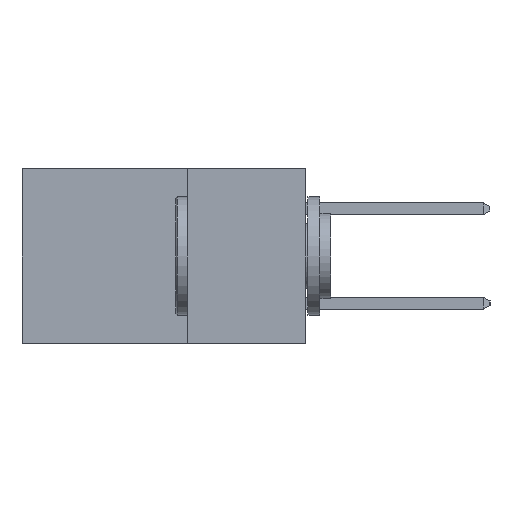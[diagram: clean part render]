
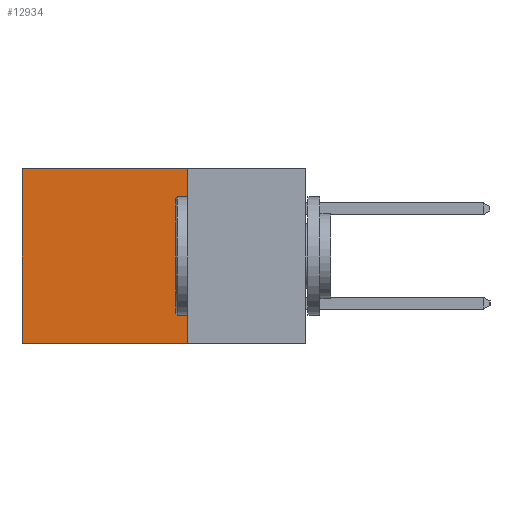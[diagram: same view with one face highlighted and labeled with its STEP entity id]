
A CAD part, left-side view. The second image highlights one B-rep face of the part: STEP entity #12934.
In plain terms, the highlighted planar face has unit normal (-1, 0, 0).
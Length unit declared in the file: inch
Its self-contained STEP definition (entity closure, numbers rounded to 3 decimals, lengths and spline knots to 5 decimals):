
#339 = EDGE_CURVE ( 'NONE', #3913, #16367, #9802, .T. ) ;
#655 = EDGE_LOOP ( 'NONE', ( #7367, #7930, #14706, #15632 ) ) ;
#988 = LINE ( 'NONE', #4701, #7487 ) ;
#1065 = PLANE ( 'NONE',  #3046 ) ;
#1839 = CARTESIAN_POINT ( 'NONE',  ( 0.2615, 0.6, -0.37 ) ) ;
#2129 = CARTESIAN_POINT ( 'NONE',  ( 0.2615, 0.25, -0.37 ) ) ;
#2332 = EDGE_CURVE ( 'NONE', #4709, #16367, #988, .T. ) ;
#2365 = LINE ( 'NONE', #2129, #15818 ) ;
#3046 = AXIS2_PLACEMENT_3D ( 'NONE', #3681, #12861, #4972 ) ;
#3083 = CARTESIAN_POINT ( 'NONE',  ( 0.2615, 0.25, -0.37 ) ) ;
#3352 = VECTOR ( 'NONE', #15177, 39.37008 ) ;
#3372 = CARTESIAN_POINT ( 'NONE',  ( 0.2615, 0.25, 0. ) ) ;
#3681 = CARTESIAN_POINT ( 'NONE',  ( 0.2615, 0.25, -0.37 ) ) ;
#3913 = VERTEX_POINT ( 'NONE', #10504 ) ;
#4384 = VERTEX_POINT ( 'NONE', #5692 ) ;
#4701 = CARTESIAN_POINT ( 'NONE',  ( 0.2615, 0.25, -0.37 ) ) ;
#4709 = VERTEX_POINT ( 'NONE', #3083 ) ;
#4972 = DIRECTION ( 'NONE',  ( 0., 0., -1. ) ) ;
#5692 = CARTESIAN_POINT ( 'NONE',  ( 0.2615, 0.25, 0. ) ) ;
#5900 = VECTOR ( 'NONE', #12902, 39.37008 ) ;
#6789 = LINE ( 'NONE', #3372, #3352 ) ;
#7367 = ORIENTED_EDGE ( 'NONE', *, *, #339, .T. ) ;
#7483 = EDGE_CURVE ( 'NONE', #4384, #3913, #6789, .T. ) ;
#7487 = VECTOR ( 'NONE', #12334, 39.37008 ) ;
#7930 = ORIENTED_EDGE ( 'NONE', *, *, #2332, .F. ) ;
#9802 = LINE ( 'NONE', #1839, #5900 ) ;
#10504 = CARTESIAN_POINT ( 'NONE',  ( 0.2615, 0.6, 0. ) ) ;
#12334 = DIRECTION ( 'NONE',  ( 0., 1., 0. ) ) ;
#12861 = DIRECTION ( 'NONE',  ( 1., 0., 0. ) ) ;
#12902 = DIRECTION ( 'NONE',  ( 0., 0., -1. ) ) ;
#12934 = ADVANCED_FACE ( 'NONE', ( #14635 ), #1065, .F. ) ;
#13883 = DIRECTION ( 'NONE',  ( 0., 0., -1. ) ) ;
#14548 = EDGE_CURVE ( 'NONE', #4384, #4709, #2365, .T. ) ;
#14635 = FACE_OUTER_BOUND ( 'NONE', #655, .T. ) ;
#14706 = ORIENTED_EDGE ( 'NONE', *, *, #14548, .F. ) ;
#15177 = DIRECTION ( 'NONE',  ( 0., 1., 0. ) ) ;
#15632 = ORIENTED_EDGE ( 'NONE', *, *, #7483, .T. ) ;
#15818 = VECTOR ( 'NONE', #13883, 39.37008 ) ;
#16101 = CARTESIAN_POINT ( 'NONE',  ( 0.2615, 0.6, -0.37 ) ) ;
#16367 = VERTEX_POINT ( 'NONE', #16101 ) ;
